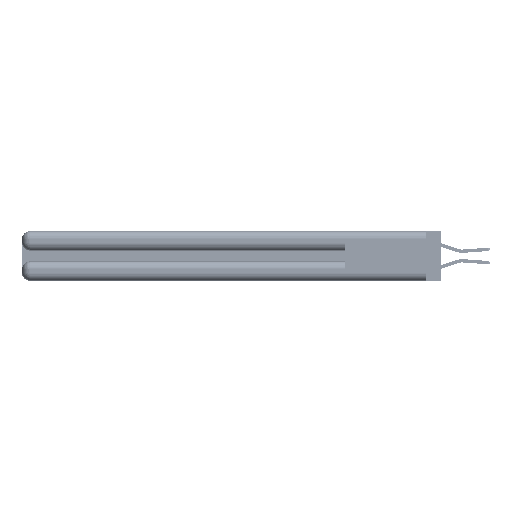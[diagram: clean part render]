
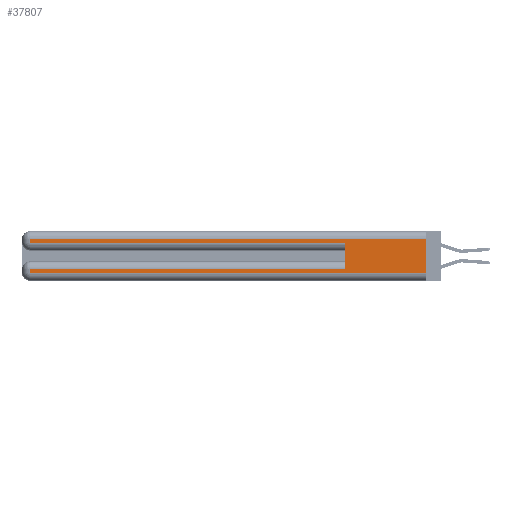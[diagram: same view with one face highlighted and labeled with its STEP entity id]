
A CAD part, left-side view. The second image highlights one B-rep face of the part: STEP entity #37807.
In plain terms, the highlighted planar face has unit normal (-1, 0, 0).
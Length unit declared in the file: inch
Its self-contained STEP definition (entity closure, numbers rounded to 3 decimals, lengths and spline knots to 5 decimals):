
#57 = VECTOR ( 'NONE', #29278, 39.37008 ) ;
#883 = EDGE_CURVE ( 'NONE', #4657, #33507, #20453, .T. ) ;
#2521 = CARTESIAN_POINT ( 'NONE',  ( 0., 0., 0.285 ) ) ;
#3721 = DIRECTION ( 'NONE',  ( 0., 0., -1. ) ) ;
#4045 = CARTESIAN_POINT ( 'NONE',  ( 0., 2.94, 0.37 ) ) ;
#4125 = CARTESIAN_POINT ( 'NONE',  ( 0., 2.94, 0.085 ) ) ;
#4657 = VERTEX_POINT ( 'NONE', #24994 ) ;
#4889 = LINE ( 'NONE', #13923, #57 ) ;
#5212 = LINE ( 'NONE', #46773, #15485 ) ;
#5886 = LINE ( 'NONE', #38577, #7096 ) ;
#7096 = VECTOR ( 'NONE', #23143, 39.37008 ) ;
#9332 = LINE ( 'NONE', #25891, #14173 ) ;
#10788 = VERTEX_POINT ( 'NONE', #39972 ) ;
#12171 = DIRECTION ( 'NONE',  ( 0., 1., 0. ) ) ;
#12524 = ORIENTED_EDGE ( 'NONE', *, *, #16818, .F. ) ;
#13250 = VECTOR ( 'NONE', #36228, 39.37008 ) ;
#13923 = CARTESIAN_POINT ( 'NONE',  ( 0., 0.6, 0.145 ) ) ;
#14173 = VECTOR ( 'NONE', #48778, 39.37008 ) ;
#14410 = CARTESIAN_POINT ( 'NONE',  ( 0., 2.94, 0.31 ) ) ;
#14913 = ORIENTED_EDGE ( 'NONE', *, *, #23338, .T. ) ;
#15485 = VECTOR ( 'NONE', #26596, 39.37008 ) ;
#15975 = VERTEX_POINT ( 'NONE', #14410 ) ;
#16818 = EDGE_CURVE ( 'NONE', #38454, #20278, #4889, .T. ) ;
#17609 = CARTESIAN_POINT ( 'NONE',  ( 0., 0., 0.06 ) ) ;
#18110 = CARTESIAN_POINT ( 'NONE',  ( 0., 0.6, 0.085 ) ) ;
#18510 = ORIENTED_EDGE ( 'NONE', *, *, #30155, .T. ) ;
#18566 = DIRECTION ( 'NONE',  ( 1., 0., 0. ) ) ;
#20202 = EDGE_CURVE ( 'NONE', #10788, #33507, #9332, .T. ) ;
#20278 = VERTEX_POINT ( 'NONE', #37749 ) ;
#20453 = LINE ( 'NONE', #17609, #13250 ) ;
#21572 = CARTESIAN_POINT ( 'NONE',  ( 0., 0., 0.06 ) ) ;
#22415 = VECTOR ( 'NONE', #49355, 39.37008 ) ;
#23143 = DIRECTION ( 'NONE',  ( 0., 1., 0. ) ) ;
#23181 = VECTOR ( 'NONE', #3721, 39.37008 ) ;
#23338 = EDGE_CURVE ( 'NONE', #42983, #4657, #38363, .T. ) ;
#24757 = EDGE_CURVE ( 'NONE', #38454, #42983, #26057, .T. ) ;
#24994 = CARTESIAN_POINT ( 'NONE',  ( 0., 2.94, 0.06 ) ) ;
#25891 = CARTESIAN_POINT ( 'NONE',  ( 0., 0., 0.37 ) ) ;
#26057 = LINE ( 'NONE', #27357, #37579 ) ;
#26596 = DIRECTION ( 'NONE',  ( 0., 0., -1. ) ) ;
#27357 = CARTESIAN_POINT ( 'NONE',  ( 0., 0., 0.085 ) ) ;
#27770 = EDGE_CURVE ( 'NONE', #10788, #15975, #5886, .T. ) ;
#28045 = EDGE_LOOP ( 'NONE', ( #44118, #41571, #18510, #45676, #12524, #30102, #14913, #36019 ) ) ;
#29278 = DIRECTION ( 'NONE',  ( 0., 0., 1. ) ) ;
#30102 = ORIENTED_EDGE ( 'NONE', *, *, #24757, .T. ) ;
#30155 = EDGE_CURVE ( 'NONE', #15975, #33171, #5212, .T. ) ;
#32009 = AXIS2_PLACEMENT_3D ( 'NONE', #41615, #18566, #44991 ) ;
#33171 = VERTEX_POINT ( 'NONE', #47029 ) ;
#33333 = LINE ( 'NONE', #2521, #22415 ) ;
#33507 = VERTEX_POINT ( 'NONE', #21572 ) ;
#33571 = EDGE_CURVE ( 'NONE', #33171, #20278, #33333, .T. ) ;
#36019 = ORIENTED_EDGE ( 'NONE', *, *, #883, .T. ) ;
#36228 = DIRECTION ( 'NONE',  ( 0., -1., 0. ) ) ;
#37579 = VECTOR ( 'NONE', #12171, 39.37008 ) ;
#37749 = CARTESIAN_POINT ( 'NONE',  ( 0., 0.6, 0.285 ) ) ;
#37807 = ADVANCED_FACE ( 'NONE', ( #47456 ), #45656, .F. ) ;
#38363 = LINE ( 'NONE', #4045, #23181 ) ;
#38454 = VERTEX_POINT ( 'NONE', #18110 ) ;
#38577 = CARTESIAN_POINT ( 'NONE',  ( 0., 0., 0.31 ) ) ;
#39972 = CARTESIAN_POINT ( 'NONE',  ( 0., 0., 0.31 ) ) ;
#41571 = ORIENTED_EDGE ( 'NONE', *, *, #27770, .T. ) ;
#41615 = CARTESIAN_POINT ( 'NONE',  ( 0., 0., 0.37 ) ) ;
#42983 = VERTEX_POINT ( 'NONE', #4125 ) ;
#44118 = ORIENTED_EDGE ( 'NONE', *, *, #20202, .F. ) ;
#44991 = DIRECTION ( 'NONE',  ( 0., 0., -1. ) ) ;
#45656 = PLANE ( 'NONE',  #32009 ) ;
#45676 = ORIENTED_EDGE ( 'NONE', *, *, #33571, .T. ) ;
#46773 = CARTESIAN_POINT ( 'NONE',  ( 0., 2.94, 0.37 ) ) ;
#47029 = CARTESIAN_POINT ( 'NONE',  ( 0., 2.94, 0.285 ) ) ;
#47456 = FACE_OUTER_BOUND ( 'NONE', #28045, .T. ) ;
#48778 = DIRECTION ( 'NONE',  ( 0., 0., -1. ) ) ;
#49355 = DIRECTION ( 'NONE',  ( 0., -1., 0. ) ) ;
